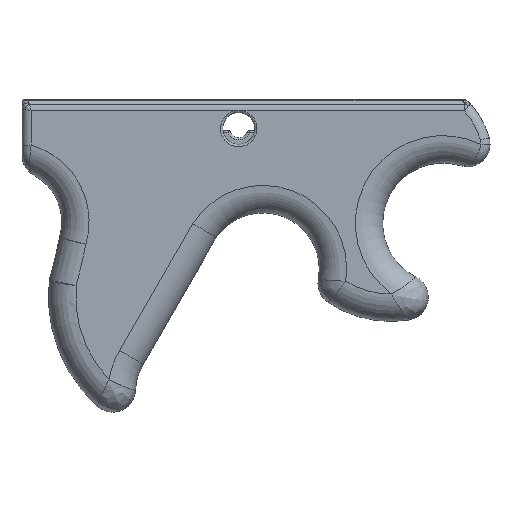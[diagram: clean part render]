
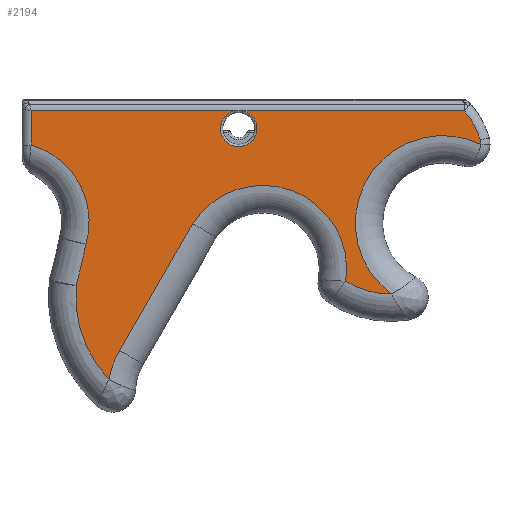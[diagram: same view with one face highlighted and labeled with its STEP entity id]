
A CAD part, top view. The second image highlights one B-rep face of the part: STEP entity #2194.
In plain terms, the highlighted planar face has unit normal (0, 0, 1).
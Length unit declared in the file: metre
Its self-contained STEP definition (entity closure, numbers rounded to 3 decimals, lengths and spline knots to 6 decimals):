
#90=CIRCLE('',#2308,0.015813);
#99=CIRCLE('',#2320,0.003);
#103=CIRCLE('',#2328,0.019221);
#109=CIRCLE('',#2338,0.018641);
#115=CIRCLE('',#2348,0.018364);
#119=CIRCLE('',#2358,0.018293);
#122=CIRCLE('',#2363,0.026212);
#129=CIRCLE('',#2375,0.159798);
#135=CIRCLE('',#2384,0.017536);
#141=CIRCLE('',#2406,0.004);
#324=LINE('',#4020,#448);
#336=LINE('',#4364,#460);
#349=LINE('',#4419,#473);
#350=LINE('',#4426,#474);
#448=VECTOR('',#2711,1.);
#460=VECTOR('',#2817,1.);
#473=VECTOR('',#2842,1.);
#474=VECTOR('',#2843,1.);
#912=ORIENTED_EDGE('',*,*,#1421,.T.);
#913=ORIENTED_EDGE('',*,*,#1434,.T.);
#914=ORIENTED_EDGE('',*,*,#1419,.T.);
#915=ORIENTED_EDGE('',*,*,#1402,.T.);
#916=ORIENTED_EDGE('',*,*,#1385,.T.);
#917=ORIENTED_EDGE('',*,*,#1374,.T.);
#918=ORIENTED_EDGE('',*,*,#1367,.T.);
#919=ORIENTED_EDGE('',*,*,#1360,.T.);
#920=ORIENTED_EDGE('',*,*,#1346,.T.);
#921=ORIENTED_EDGE('',*,*,#1344,.T.);
#922=ORIENTED_EDGE('',*,*,#1333,.T.);
#923=ORIENTED_EDGE('',*,*,#1320,.T.);
#924=ORIENTED_EDGE('',*,*,#1309,.T.);
#925=ORIENTED_EDGE('',*,*,#1300,.T.);
#1300=EDGE_CURVE('',#1617,#1616,#90,.T.);
#1309=EDGE_CURVE('',#1621,#1617,#99,.T.);
#1320=EDGE_CURVE('',#1628,#1621,#103,.F.);
#1333=EDGE_CURVE('',#1634,#1628,#109,.T.);
#1344=EDGE_CURVE('',#1640,#1634,#115,.F.);
#1346=EDGE_CURVE('',#1641,#1640,#324,.F.);
#1360=EDGE_CURVE('',#1650,#1641,#119,.F.);
#1367=EDGE_CURVE('',#1610,#1650,#122,.T.);
#1374=EDGE_CURVE('',#1609,#1610,#129,.F.);
#1385=EDGE_CURVE('',#1659,#1609,#135,.F.);
#1402=EDGE_CURVE('',#1667,#1659,#336,.F.);
#1419=EDGE_CURVE('',#1679,#1667,#349,.F.);
#1421=EDGE_CURVE('',#1616,#1680,#350,.F.);
#1434=EDGE_CURVE('',#1680,#1679,#141,.F.);
#1609=VERTEX_POINT('',#3480);
#1610=VERTEX_POINT('',#3511);
#1616=VERTEX_POINT('',#3621);
#1617=VERTEX_POINT('',#3628);
#1621=VERTEX_POINT('',#3642);
#1628=VERTEX_POINT('',#3753);
#1634=VERTEX_POINT('',#3929);
#1640=VERTEX_POINT('',#4012);
#1641=VERTEX_POINT('',#4021);
#1650=VERTEX_POINT('',#4066);
#1659=VERTEX_POINT('',#4268);
#1667=VERTEX_POINT('',#4365);
#1679=VERTEX_POINT('',#4420);
#1680=VERTEX_POINT('',#4425);
#1881=EDGE_LOOP('',(#912,#913,#914,#915,#916,#917,#918,#919,#920,#921,#922,
#923,#924,#925));
#2022=FACE_BOUND('',#1881,.T.);
#2088=PLANE('',#2405);
#2194=ADVANCED_FACE('',(#2022),#2088,.T.);
#2308=AXIS2_PLACEMENT_3D('',#3627,#2621,#2622);
#2320=AXIS2_PLACEMENT_3D('',#3645,#2645,#2646);
#2328=AXIS2_PLACEMENT_3D('',#3752,#2663,#2664);
#2338=AXIS2_PLACEMENT_3D('',#3930,#2685,#2686);
#2348=AXIS2_PLACEMENT_3D('',#4011,#2707,#2708);
#2358=AXIS2_PLACEMENT_3D('',#4065,#2733,#2734);
#2363=AXIS2_PLACEMENT_3D('',#4188,#2744,#2745);
#2375=AXIS2_PLACEMENT_3D('',#4200,#2768,#2769);
#2384=AXIS2_PLACEMENT_3D('',#4267,#2787,#2788);
#2405=AXIS2_PLACEMENT_3D('',#4463,#2856,#2857);
#2406=AXIS2_PLACEMENT_3D('',#4464,#2858,#2859);
#2621=DIRECTION('',(0.,0.,1.));
#2622=DIRECTION('',(1.,0.,0.));
#2645=DIRECTION('',(0.,0.,1.));
#2646=DIRECTION('',(1.,0.,0.));
#2663=DIRECTION('',(0.,0.,1.));
#2664=DIRECTION('',(1.,0.,0.));
#2685=DIRECTION('',(0.,0.,1.));
#2686=DIRECTION('',(1.,0.,0.));
#2707=DIRECTION('',(0.,0.,1.));
#2708=DIRECTION('',(1.,0.,0.));
#2711=DIRECTION('',(-0.5,-0.866,0.));
#2733=DIRECTION('',(0.,0.,1.));
#2734=DIRECTION('',(1.,0.,0.));
#2744=DIRECTION('',(0.,0.,1.));
#2745=DIRECTION('',(1.,0.,0.));
#2768=DIRECTION('',(0.,0.,1.));
#2769=DIRECTION('',(1.,0.,0.));
#2787=DIRECTION('',(0.,0.,1.));
#2788=DIRECTION('',(1.,0.,0.));
#2817=DIRECTION('',(0.,1.,0.));
#2842=DIRECTION('',(1.,0.,0.));
#2843=DIRECTION('',(1.,0.,0.));
#2856=DIRECTION('',(0.,0.,1.));
#2857=DIRECTION('',(1.,0.,0.));
#2858=DIRECTION('',(0.,0.,1.));
#2859=DIRECTION('',(1.,0.,0.));
#3480=CARTESIAN_POINT('',(-0.03837,-0.005522,0.026));
#3511=CARTESIAN_POINT('',(-0.040498,-0.014616,0.026));
#3621=CARTESIAN_POINT('',(0.044705,0.023775,0.026));
#3627=CARTESIAN_POINT('',(0.033005,0.013138,0.026));
#3628=CARTESIAN_POINT('',(0.048253,0.017326,0.026));
#3642=CARTESIAN_POINT('',(0.048359,0.016428,0.026));
#3645=CARTESIAN_POINT('',(0.04536,0.016531,0.026));
#3752=CARTESIAN_POINT('',(0.040016,-0.000889,0.026));
#3753=CARTESIAN_POINT('',(0.028715,-0.016437,0.026));
#3929=CARTESIAN_POINT('',(0.018681,-0.013622,0.026));
#3930=CARTESIAN_POINT('',(0.028532,0.002203,0.026));
#4011=CARTESIAN_POINT('',(0.000511,-0.01096,0.026));
#4012=CARTESIAN_POINT('',(-0.014882,-0.000945,0.026));
#4020=CARTESIAN_POINT('',(-0.007176,0.012412,0.026));
#4021=CARTESIAN_POINT('',(-0.030975,-0.02884,0.026));
#4065=CARTESIAN_POINT('',(-0.015221,-0.038137,0.026));
#4066=CARTESIAN_POINT('',(-0.033278,-0.03521,0.026));
#4188=CARTESIAN_POINT('',(-0.014398,-0.017028,0.026));
#4200=CARTESIAN_POINT('',(-0.194963,0.026323,0.026));
#4267=CARTESIAN_POINT('',(-0.0552,-0.000594,0.026));
#4268=CARTESIAN_POINT('',(-0.050396,0.016271,0.026));
#4364=CARTESIAN_POINT('',(-0.050396,0.003343,0.026));
#4365=CARTESIAN_POINT('',(-0.050396,0.023775,0.026));
#4419=CARTESIAN_POINT('',(0.008544,0.023775,0.026));
#4420=CARTESIAN_POINT('',(-0.005773,0.023775,0.026));
#4425=CARTESIAN_POINT('',(-0.003875,0.023775,0.026));
#4426=CARTESIAN_POINT('',(0.008544,0.023775,0.026));
#4463=CARTESIAN_POINT('',(0.008544,0.003343,0.026));
#4464=CARTESIAN_POINT('',(-0.004824,0.019889,0.026));
